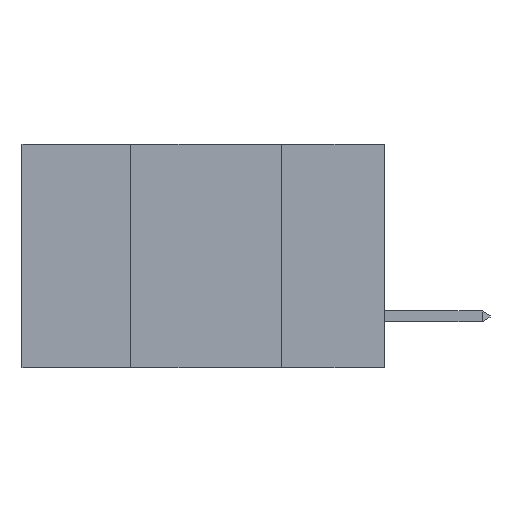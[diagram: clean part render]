
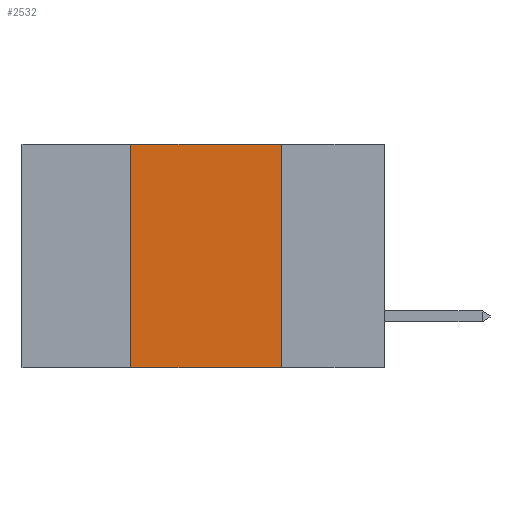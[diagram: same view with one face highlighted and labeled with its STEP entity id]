
A CAD part, left-side view. The second image highlights one B-rep face of the part: STEP entity #2532.
In plain terms, the highlighted planar face has unit normal (-1, 0, 0).
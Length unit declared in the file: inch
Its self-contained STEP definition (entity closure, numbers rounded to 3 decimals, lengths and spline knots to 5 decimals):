
#230 = VECTOR ( 'NONE', #11935, 39.37008 ) ;
#274 = CARTESIAN_POINT ( 'NONE',  ( 0., 0.17, 0. ) ) ;
#306 = EDGE_CURVE ( 'NONE', #6401, #6059, #12466, .T. ) ;
#372 = CARTESIAN_POINT ( 'NONE',  ( 0., 0.42, 0. ) ) ;
#377 = ORIENTED_EDGE ( 'NONE', *, *, #11615, .F. ) ;
#519 = ORIENTED_EDGE ( 'NONE', *, *, #306, .T. ) ;
#622 = DIRECTION ( 'NONE',  ( 0., -1., 0. ) ) ;
#762 = CARTESIAN_POINT ( 'NONE',  ( 0., 0.17, -0.37 ) ) ;
#1012 = ORIENTED_EDGE ( 'NONE', *, *, #6336, .F. ) ;
#1208 = ORIENTED_EDGE ( 'NONE', *, *, #10245, .F. ) ;
#1214 = CARTESIAN_POINT ( 'NONE',  ( 0., 0.17, 0. ) ) ;
#1792 = LINE ( 'NONE', #274, #9732 ) ;
#1910 = AXIS2_PLACEMENT_3D ( 'NONE', #11795, #9295, #2718 ) ;
#2532 = ADVANCED_FACE ( 'NONE', ( #3410 ), #12040, .F. ) ;
#2718 = DIRECTION ( 'NONE',  ( 0., 0., -1. ) ) ;
#2761 = CARTESIAN_POINT ( 'NONE',  ( 0., 0.42, 0. ) ) ;
#2976 = LINE ( 'NONE', #7089, #230 ) ;
#3336 = DIRECTION ( 'NONE',  ( 0., 0., -1. ) ) ;
#3410 = FACE_OUTER_BOUND ( 'NONE', #11596, .T. ) ;
#4307 = CARTESIAN_POINT ( 'NONE',  ( 0., 0.42, -0.37 ) ) ;
#6059 = VERTEX_POINT ( 'NONE', #762 ) ;
#6336 = EDGE_CURVE ( 'NONE', #12426, #6351, #2976, .T. ) ;
#6351 = VERTEX_POINT ( 'NONE', #1214 ) ;
#6401 = VERTEX_POINT ( 'NONE', #4307 ) ;
#7089 = CARTESIAN_POINT ( 'NONE',  ( 0., 0.6, 0. ) ) ;
#7418 = VECTOR ( 'NONE', #622, 39.37008 ) ;
#8093 = CARTESIAN_POINT ( 'NONE',  ( 0., 0.6, -0.37 ) ) ;
#9295 = DIRECTION ( 'NONE',  ( 1., 0., 0. ) ) ;
#9689 = DIRECTION ( 'NONE',  ( 0., 0., 1. ) ) ;
#9732 = VECTOR ( 'NONE', #3336, 39.37008 ) ;
#9843 = LINE ( 'NONE', #2761, #11978 ) ;
#10245 = EDGE_CURVE ( 'NONE', #6351, #6059, #1792, .T. ) ;
#11596 = EDGE_LOOP ( 'NONE', ( #1208, #1012, #377, #519 ) ) ;
#11615 = EDGE_CURVE ( 'NONE', #6401, #12426, #9843, .T. ) ;
#11795 = CARTESIAN_POINT ( 'NONE',  ( 0., 0.6, 0. ) ) ;
#11935 = DIRECTION ( 'NONE',  ( 0., -1., 0. ) ) ;
#11978 = VECTOR ( 'NONE', #9689, 39.37008 ) ;
#12040 = PLANE ( 'NONE',  #1910 ) ;
#12426 = VERTEX_POINT ( 'NONE', #372 ) ;
#12466 = LINE ( 'NONE', #8093, #7418 ) ;
